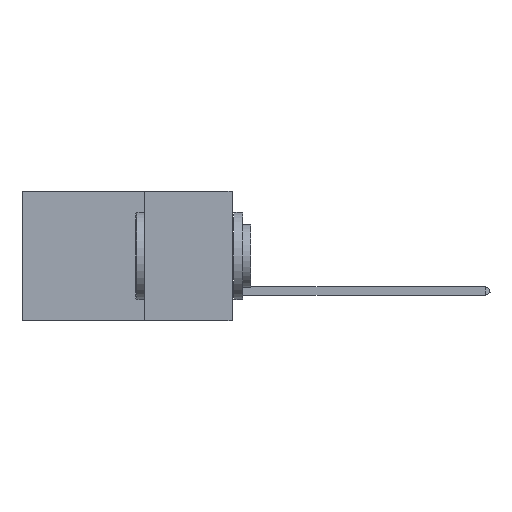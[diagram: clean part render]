
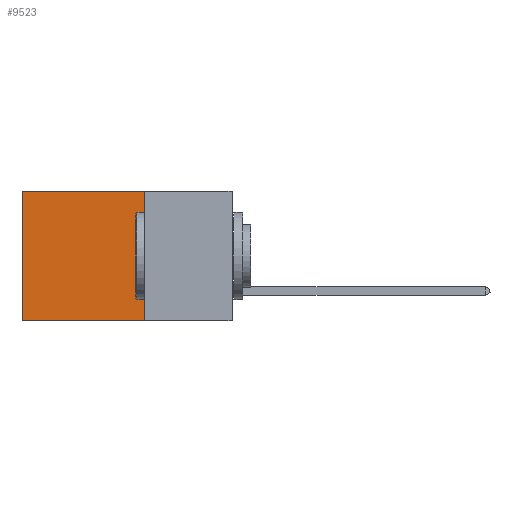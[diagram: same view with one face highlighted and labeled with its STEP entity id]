
A CAD part, left-side view. The second image highlights one B-rep face of the part: STEP entity #9523.
In plain terms, the highlighted planar face has unit normal (-1, 0, 0).
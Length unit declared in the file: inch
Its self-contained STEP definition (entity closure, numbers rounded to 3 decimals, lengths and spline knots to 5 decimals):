
#445 = DIRECTION ( 'NONE',  ( 0., 0., -1. ) ) ;
#506 = CARTESIAN_POINT ( 'NONE',  ( 0.2875, 0.6, 0. ) ) ;
#1204 = ORIENTED_EDGE ( 'NONE', *, *, #18294, .T. ) ;
#2628 = VECTOR ( 'NONE', #3727, 39.37008 ) ;
#2705 = DIRECTION ( 'NONE',  ( 0., 1., 0. ) ) ;
#2909 = CARTESIAN_POINT ( 'NONE',  ( 0.2875, 0.6, -0.37 ) ) ;
#3585 = EDGE_LOOP ( 'NONE', ( #6483, #15307, #19199, #1204 ) ) ;
#3626 = EDGE_CURVE ( 'NONE', #18616, #12763, #3895, .T. ) ;
#3727 = DIRECTION ( 'NONE',  ( 0., 0., -1. ) ) ;
#3895 = LINE ( 'NONE', #506, #11384 ) ;
#4181 = CARTESIAN_POINT ( 'NONE',  ( 0.2875, 0.25, 0. ) ) ;
#4247 = PLANE ( 'NONE',  #16960 ) ;
#5064 = CARTESIAN_POINT ( 'NONE',  ( 0.2875, 0.25, 0. ) ) ;
#5373 = DIRECTION ( 'NONE',  ( 0., 1., 0. ) ) ;
#5527 = LINE ( 'NONE', #6282, #8119 ) ;
#6090 = LINE ( 'NONE', #19079, #18205 ) ;
#6282 = CARTESIAN_POINT ( 'NONE',  ( 0.2875, 0.25, -0.37 ) ) ;
#6483 = ORIENTED_EDGE ( 'NONE', *, *, #3626, .T. ) ;
#6769 = CARTESIAN_POINT ( 'NONE',  ( 0.2875, 0.6, 0. ) ) ;
#6874 = DIRECTION ( 'NONE',  ( 0., 0., -1. ) ) ;
#6975 = CARTESIAN_POINT ( 'NONE',  ( 0.2875, 0.25, -0.37 ) ) ;
#8119 = VECTOR ( 'NONE', #5373, 39.37008 ) ;
#8231 = FACE_OUTER_BOUND ( 'NONE', #3585, .T. ) ;
#9523 = ADVANCED_FACE ( 'NONE', ( #8231 ), #4247, .F. ) ;
#11296 = DIRECTION ( 'NONE',  ( 1., 0., 0. ) ) ;
#11384 = VECTOR ( 'NONE', #445, 39.37008 ) ;
#12118 = EDGE_CURVE ( 'NONE', #14934, #12763, #5527, .T. ) ;
#12763 = VERTEX_POINT ( 'NONE', #2909 ) ;
#13375 = LINE ( 'NONE', #18604, #2628 ) ;
#13586 = EDGE_CURVE ( 'NONE', #15845, #14934, #13375, .T. ) ;
#14934 = VERTEX_POINT ( 'NONE', #6975 ) ;
#15307 = ORIENTED_EDGE ( 'NONE', *, *, #12118, .F. ) ;
#15845 = VERTEX_POINT ( 'NONE', #5064 ) ;
#16960 = AXIS2_PLACEMENT_3D ( 'NONE', #4181, #11296, #6874 ) ;
#18205 = VECTOR ( 'NONE', #2705, 39.37008 ) ;
#18294 = EDGE_CURVE ( 'NONE', #15845, #18616, #6090, .T. ) ;
#18604 = CARTESIAN_POINT ( 'NONE',  ( 0.2875, 0.25, 0. ) ) ;
#18616 = VERTEX_POINT ( 'NONE', #6769 ) ;
#19079 = CARTESIAN_POINT ( 'NONE',  ( 0.2875, 0.25, 0. ) ) ;
#19199 = ORIENTED_EDGE ( 'NONE', *, *, #13586, .F. ) ;
